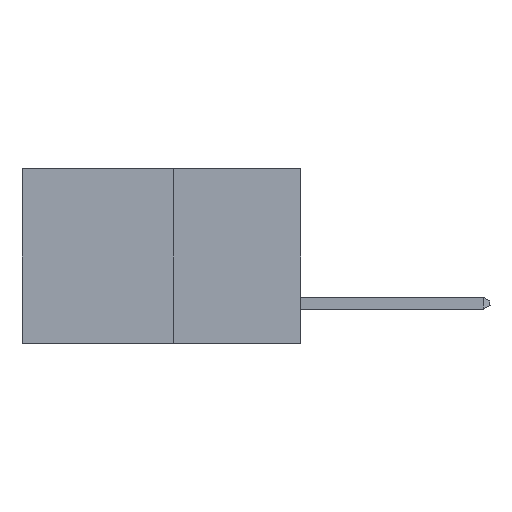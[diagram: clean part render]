
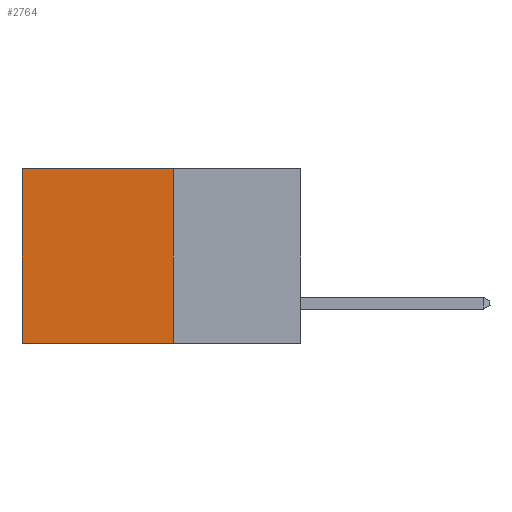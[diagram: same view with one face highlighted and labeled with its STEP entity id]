
A CAD part, left-side view. The second image highlights one B-rep face of the part: STEP entity #2764.
In plain terms, the highlighted planar face has unit normal (-1, 0, 0).
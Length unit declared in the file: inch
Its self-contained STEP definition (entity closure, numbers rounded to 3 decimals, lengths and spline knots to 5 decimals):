
#283 = VERTEX_POINT ( 'NONE', #18184 ) ;
#1955 = CARTESIAN_POINT ( 'NONE',  ( 0.277, 0.59, 0. ) ) ;
#2078 = PLANE ( 'NONE',  #6239 ) ;
#2421 = CARTESIAN_POINT ( 'NONE',  ( 0.277, 0.27, -0.37 ) ) ;
#2764 = ADVANCED_FACE ( 'NONE', ( #24422 ), #2078, .F. ) ;
#3664 = CARTESIAN_POINT ( 'NONE',  ( 0.277, 0.27, 0. ) ) ;
#5844 = LINE ( 'NONE', #15878, #16981 ) ;
#6239 = AXIS2_PLACEMENT_3D ( 'NONE', #8794, #24326, #10996 ) ;
#7819 = CARTESIAN_POINT ( 'NONE',  ( 0.277, 0.27, -0.37 ) ) ;
#8731 = LINE ( 'NONE', #7819, #18481 ) ;
#8794 = CARTESIAN_POINT ( 'NONE',  ( 0.277, 0.27, -0.37 ) ) ;
#9592 = EDGE_CURVE ( 'NONE', #20244, #11367, #12381, .T. ) ;
#10996 = DIRECTION ( 'NONE',  ( 0., 0., -1. ) ) ;
#11367 = VERTEX_POINT ( 'NONE', #2421 ) ;
#11674 = VECTOR ( 'NONE', #26677, 39.37008 ) ;
#12050 = CARTESIAN_POINT ( 'NONE',  ( 0.277, 0.59, -0.37 ) ) ;
#12371 = EDGE_CURVE ( 'NONE', #11367, #283, #8731, .T. ) ;
#12381 = LINE ( 'NONE', #20057, #11674 ) ;
#12440 = ORIENTED_EDGE ( 'NONE', *, *, #9592, .F. ) ;
#14393 = EDGE_CURVE ( 'NONE', #15953, #283, #26583, .T. ) ;
#15878 = CARTESIAN_POINT ( 'NONE',  ( 0.277, 0.27, 0. ) ) ;
#15953 = VERTEX_POINT ( 'NONE', #1955 ) ;
#16100 = ORIENTED_EDGE ( 'NONE', *, *, #14393, .T. ) ;
#16981 = VECTOR ( 'NONE', #24715, 39.37008 ) ;
#17417 = ORIENTED_EDGE ( 'NONE', *, *, #19224, .T. ) ;
#18184 = CARTESIAN_POINT ( 'NONE',  ( 0.277, 0.59, -0.37 ) ) ;
#18481 = VECTOR ( 'NONE', #27743, 39.37008 ) ;
#18644 = ORIENTED_EDGE ( 'NONE', *, *, #12371, .F. ) ;
#19224 = EDGE_CURVE ( 'NONE', #20244, #15953, #5844, .T. ) ;
#20057 = CARTESIAN_POINT ( 'NONE',  ( 0.277, 0.27, -0.37 ) ) ;
#20244 = VERTEX_POINT ( 'NONE', #3664 ) ;
#22122 = VECTOR ( 'NONE', #25339, 39.37008 ) ;
#23288 = EDGE_LOOP ( 'NONE', ( #16100, #18644, #12440, #17417 ) ) ;
#24326 = DIRECTION ( 'NONE',  ( 1., 0., 0. ) ) ;
#24422 = FACE_OUTER_BOUND ( 'NONE', #23288, .T. ) ;
#24715 = DIRECTION ( 'NONE',  ( 0., 1., 0. ) ) ;
#25339 = DIRECTION ( 'NONE',  ( 0., 0., -1. ) ) ;
#26583 = LINE ( 'NONE', #12050, #22122 ) ;
#26677 = DIRECTION ( 'NONE',  ( 0., 0., -1. ) ) ;
#27743 = DIRECTION ( 'NONE',  ( 0., 1., 0. ) ) ;
